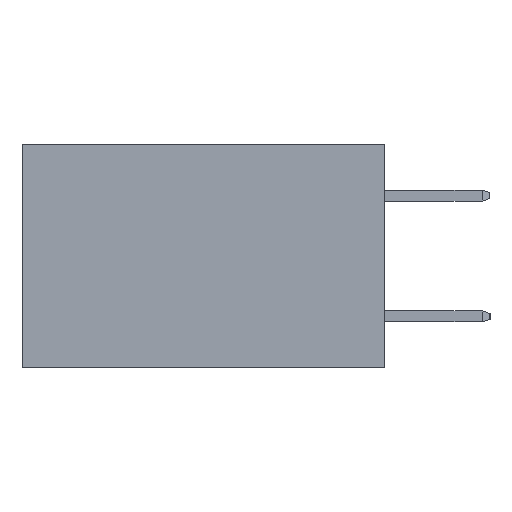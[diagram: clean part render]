
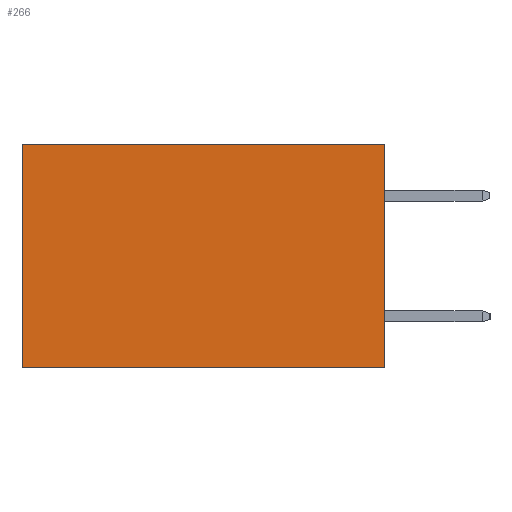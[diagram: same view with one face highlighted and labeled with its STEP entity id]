
A CAD part, left-side view. The second image highlights one B-rep face of the part: STEP entity #266.
In plain terms, the highlighted planar face has unit normal (-1, 0, 0).
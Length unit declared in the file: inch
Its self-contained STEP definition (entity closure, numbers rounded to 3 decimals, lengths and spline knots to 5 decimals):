
#266 = ADVANCED_FACE ( 'NONE', ( #9798 ), #464, .F. ) ;
#334 = DIRECTION ( 'NONE',  ( 1., 0., 0. ) ) ;
#464 = PLANE ( 'NONE',  #5186 ) ;
#579 = DIRECTION ( 'NONE',  ( 0., 0., -1. ) ) ;
#688 = DIRECTION ( 'NONE',  ( 0., 0., -1. ) ) ;
#1043 = CARTESIAN_POINT ( 'NONE',  ( 0.2615, 0.6, 0. ) ) ;
#1181 = CARTESIAN_POINT ( 'NONE',  ( 0.2615, 0., 0. ) ) ;
#1493 = CARTESIAN_POINT ( 'NONE',  ( 0.2615, 0., -0.37 ) ) ;
#2738 = CARTESIAN_POINT ( 'NONE',  ( 0.2615, 0.6, -0.37 ) ) ;
#2796 = VECTOR ( 'NONE', #9834, 39.37008 ) ;
#3274 = VECTOR ( 'NONE', #7758, 39.37008 ) ;
#3748 = CARTESIAN_POINT ( 'NONE',  ( 0.2615, 0., 0. ) ) ;
#3774 = DIRECTION ( 'NONE',  ( 0., 1., 0. ) ) ;
#3822 = CARTESIAN_POINT ( 'NONE',  ( 0.2615, 0.6, -0.37 ) ) ;
#4101 = VECTOR ( 'NONE', #3774, 39.37008 ) ;
#4759 = CARTESIAN_POINT ( 'NONE',  ( 0.2615, 0., -0.37 ) ) ;
#5186 = AXIS2_PLACEMENT_3D ( 'NONE', #1493, #334, #579 ) ;
#5219 = ORIENTED_EDGE ( 'NONE', *, *, #12194, .F. ) ;
#6026 = VERTEX_POINT ( 'NONE', #10377 ) ;
#6087 = ORIENTED_EDGE ( 'NONE', *, *, #6627, .T. ) ;
#6495 = VECTOR ( 'NONE', #688, 39.37008 ) ;
#6627 = EDGE_CURVE ( 'NONE', #12310, #6789, #6974, .T. ) ;
#6789 = VERTEX_POINT ( 'NONE', #1043 ) ;
#6974 = LINE ( 'NONE', #3748, #4101 ) ;
#7282 = EDGE_LOOP ( 'NONE', ( #12753, #5219, #11103, #6087 ) ) ;
#7758 = DIRECTION ( 'NONE',  ( 0., 0., -1. ) ) ;
#8075 = LINE ( 'NONE', #8854, #2796 ) ;
#8854 = CARTESIAN_POINT ( 'NONE',  ( 0.2615, 0., -0.37 ) ) ;
#9121 = LINE ( 'NONE', #4759, #6495 ) ;
#9798 = FACE_OUTER_BOUND ( 'NONE', #7282, .T. ) ;
#9834 = DIRECTION ( 'NONE',  ( 0., 1., 0. ) ) ;
#10377 = CARTESIAN_POINT ( 'NONE',  ( 0.2615, 0., -0.37 ) ) ;
#11103 = ORIENTED_EDGE ( 'NONE', *, *, #12699, .F. ) ;
#11515 = LINE ( 'NONE', #3822, #3274 ) ;
#12194 = EDGE_CURVE ( 'NONE', #6026, #12723, #8075, .T. ) ;
#12310 = VERTEX_POINT ( 'NONE', #1181 ) ;
#12699 = EDGE_CURVE ( 'NONE', #12310, #6026, #9121, .T. ) ;
#12723 = VERTEX_POINT ( 'NONE', #2738 ) ;
#12753 = ORIENTED_EDGE ( 'NONE', *, *, #12758, .T. ) ;
#12758 = EDGE_CURVE ( 'NONE', #6789, #12723, #11515, .T. ) ;
